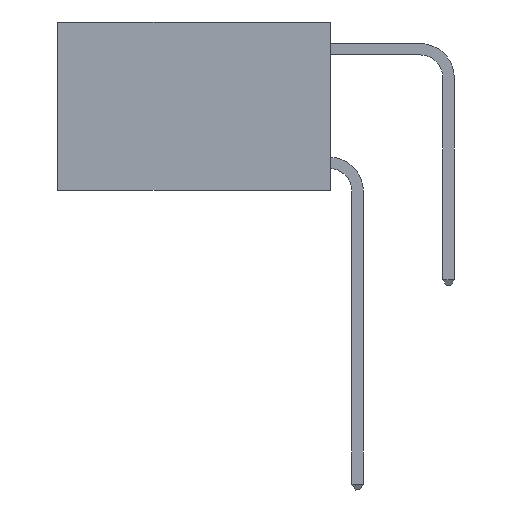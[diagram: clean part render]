
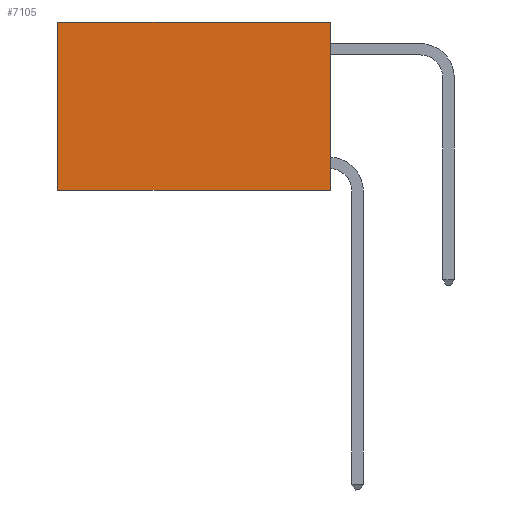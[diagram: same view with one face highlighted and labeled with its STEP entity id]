
A CAD part, left-side view. The second image highlights one B-rep face of the part: STEP entity #7105.
In plain terms, the highlighted planar face has unit normal (-1, 0, 0).
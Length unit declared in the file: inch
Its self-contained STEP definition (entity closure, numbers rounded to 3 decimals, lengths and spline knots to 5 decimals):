
#544 = CARTESIAN_POINT ( 'NONE',  ( 0.2625, 0., 0. ) ) ;
#958 = CARTESIAN_POINT ( 'NONE',  ( 0.2625, 0.6, 0. ) ) ;
#1197 = DIRECTION ( 'NONE',  ( 0., 0., -1. ) ) ;
#1395 = EDGE_LOOP ( 'NONE', ( #4040, #8496, #7784, #7038 ) ) ;
#1467 = CARTESIAN_POINT ( 'NONE',  ( 0.2625, 0., -0.37 ) ) ;
#1715 = CARTESIAN_POINT ( 'NONE',  ( 0.2625, 0., 0. ) ) ;
#2081 = DIRECTION ( 'NONE',  ( 1., 0., 0. ) ) ;
#2211 = CARTESIAN_POINT ( 'NONE',  ( 0.2625, 0., -0.37 ) ) ;
#2344 = VECTOR ( 'NONE', #8226, 39.37008 ) ;
#2549 = EDGE_CURVE ( 'NONE', #2654, #6737, #7465, .T. ) ;
#2654 = VERTEX_POINT ( 'NONE', #1715 ) ;
#2711 = FACE_OUTER_BOUND ( 'NONE', #1395, .T. ) ;
#2762 = DIRECTION ( 'NONE',  ( 0., 0., -1. ) ) ;
#2832 = EDGE_CURVE ( 'NONE', #6737, #3450, #8277, .T. ) ;
#3301 = VECTOR ( 'NONE', #4496, 39.37008 ) ;
#3331 = VERTEX_POINT ( 'NONE', #958 ) ;
#3450 = VERTEX_POINT ( 'NONE', #3699 ) ;
#3699 = CARTESIAN_POINT ( 'NONE',  ( 0.2625, 0.6, -0.37 ) ) ;
#4040 = ORIENTED_EDGE ( 'NONE', *, *, #7097, .T. ) ;
#4137 = AXIS2_PLACEMENT_3D ( 'NONE', #544, #2081, #1197 ) ;
#4496 = DIRECTION ( 'NONE',  ( 0., 0., -1. ) ) ;
#5040 = CARTESIAN_POINT ( 'NONE',  ( 0.2625, 0.6, 0. ) ) ;
#5049 = EDGE_CURVE ( 'NONE', #2654, #3331, #5202, .T. ) ;
#5202 = LINE ( 'NONE', #6702, #6311 ) ;
#5953 = CARTESIAN_POINT ( 'NONE',  ( 0.2625, 0., 0. ) ) ;
#6311 = VECTOR ( 'NONE', #9009, 39.37008 ) ;
#6422 = LINE ( 'NONE', #5040, #8402 ) ;
#6702 = CARTESIAN_POINT ( 'NONE',  ( 0.2625, 0., 0. ) ) ;
#6737 = VERTEX_POINT ( 'NONE', #1467 ) ;
#7038 = ORIENTED_EDGE ( 'NONE', *, *, #5049, .T. ) ;
#7097 = EDGE_CURVE ( 'NONE', #3331, #3450, #6422, .T. ) ;
#7105 = ADVANCED_FACE ( 'NONE', ( #2711 ), #7327, .F. ) ;
#7327 = PLANE ( 'NONE',  #4137 ) ;
#7465 = LINE ( 'NONE', #5953, #3301 ) ;
#7784 = ORIENTED_EDGE ( 'NONE', *, *, #2549, .F. ) ;
#8226 = DIRECTION ( 'NONE',  ( 0., 1., 0. ) ) ;
#8277 = LINE ( 'NONE', #2211, #2344 ) ;
#8402 = VECTOR ( 'NONE', #2762, 39.37008 ) ;
#8496 = ORIENTED_EDGE ( 'NONE', *, *, #2832, .F. ) ;
#9009 = DIRECTION ( 'NONE',  ( 0., 1., 0. ) ) ;
